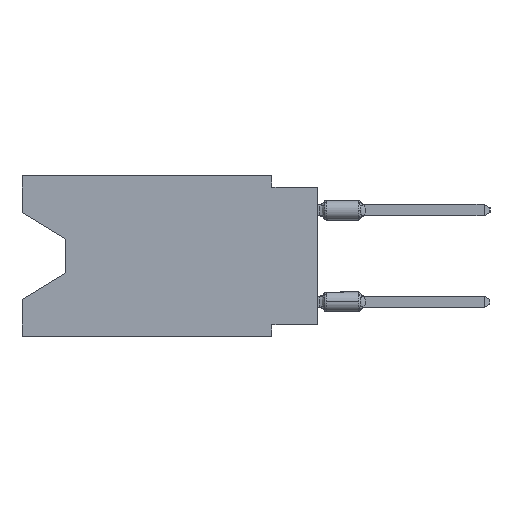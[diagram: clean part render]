
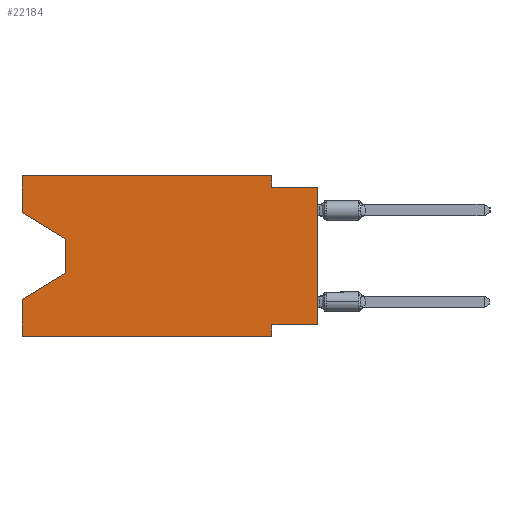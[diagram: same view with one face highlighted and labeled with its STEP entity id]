
A CAD part, left-side view. The second image highlights one B-rep face of the part: STEP entity #22184.
In plain terms, the highlighted planar face has unit normal (-1, 0, 0).
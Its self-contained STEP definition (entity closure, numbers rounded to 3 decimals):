
#291 = VECTOR ( 'NONE', #18357, 1000. ) ;
#392 = VERTEX_POINT ( 'NONE', #48890 ) ;
#420 = CARTESIAN_POINT ( 'NONE',  ( 0., 16.383, -2.038 ) ) ;
#516 = CARTESIAN_POINT ( 'NONE',  ( 0., 2.54, -8.255 ) ) ;
#1358 = EDGE_CURVE ( 'NONE', #392, #31829, #39594, .T. ) ;
#1499 = CARTESIAN_POINT ( 'NONE',  ( 0., 16.383, 0. ) ) ;
#1852 = VECTOR ( 'NONE', #46630, 1000. ) ;
#2166 = CARTESIAN_POINT ( 'NONE',  ( 0., 2.54, -8.89 ) ) ;
#2721 = CARTESIAN_POINT ( 'NONE',  ( 0., 2.54, -8.89 ) ) ;
#3894 = ORIENTED_EDGE ( 'NONE', *, *, #35941, .T. ) ;
#3950 = VECTOR ( 'NONE', #14837, 1000. ) ;
#4140 = CARTESIAN_POINT ( 'NONE',  ( 0., 16.383, 0. ) ) ;
#4143 = CARTESIAN_POINT ( 'NONE',  ( 0., 2.54, 0. ) ) ;
#4407 = CARTESIAN_POINT ( 'NONE',  ( 0., 13.97, -3.505 ) ) ;
#5212 = VECTOR ( 'NONE', #20302, 1000. ) ;
#6039 = DIRECTION ( 'NONE',  ( 0., -1., 0. ) ) ;
#6327 = VERTEX_POINT ( 'NONE', #11023 ) ;
#6406 = CARTESIAN_POINT ( 'NONE',  ( 0., 16.383, -2.038 ) ) ;
#7091 = VECTOR ( 'NONE', #18451, 1000. ) ;
#7501 = EDGE_CURVE ( 'NONE', #31712, #48774, #38444, .T. ) ;
#8876 = VECTOR ( 'NONE', #15474, 1000. ) ;
#8938 = VECTOR ( 'NONE', #41176, 1000. ) ;
#9116 = ORIENTED_EDGE ( 'NONE', *, *, #29129, .T. ) ;
#11023 = CARTESIAN_POINT ( 'NONE',  ( 0., 0., -0.635 ) ) ;
#11464 = FACE_OUTER_BOUND ( 'NONE', #32385, .T. ) ;
#12868 = ORIENTED_EDGE ( 'NONE', *, *, #27389, .T. ) ;
#14200 = CARTESIAN_POINT ( 'NONE',  ( 0., 16.383, 0. ) ) ;
#14381 = LINE ( 'NONE', #41994, #31483 ) ;
#14837 = DIRECTION ( 'NONE',  ( 0., 0., 1. ) ) ;
#15474 = DIRECTION ( 'NONE',  ( 0., 0., -1. ) ) ;
#15889 = DIRECTION ( 'NONE',  ( 1., 0., 0. ) ) ;
#16525 = LINE ( 'NONE', #43897, #22149 ) ;
#16985 = EDGE_CURVE ( 'NONE', #49438, #6327, #14381, .T. ) ;
#17812 = ORIENTED_EDGE ( 'NONE', *, *, #1358, .T. ) ;
#18153 = AXIS2_PLACEMENT_3D ( 'NONE', #4140, #15889, #27371 ) ;
#18357 = DIRECTION ( 'NONE',  ( 0., 0., 1. ) ) ;
#18451 = DIRECTION ( 'NONE',  ( 0., 0., 1. ) ) ;
#18875 = VECTOR ( 'NONE', #50354, 1000. ) ;
#19041 = CARTESIAN_POINT ( 'NONE',  ( 0., 16.383, 0. ) ) ;
#19910 = VERTEX_POINT ( 'NONE', #6406 ) ;
#20302 = DIRECTION ( 'NONE',  ( 0., 0., -1. ) ) ;
#20479 = DIRECTION ( 'NONE',  ( 0., -0.855, -0.519 ) ) ;
#21604 = LINE ( 'NONE', #29696, #8938 ) ;
#22149 = VECTOR ( 'NONE', #40761, 1000. ) ;
#22184 = ADVANCED_FACE ( 'NONE', ( #11464 ), #31798, .F. ) ;
#22480 = ORIENTED_EDGE ( 'NONE', *, *, #46277, .F. ) ;
#22631 = ORIENTED_EDGE ( 'NONE', *, *, #28700, .F. ) ;
#22652 = ORIENTED_EDGE ( 'NONE', *, *, #16985, .F. ) ;
#24172 = CARTESIAN_POINT ( 'NONE',  ( 0., 16.383, -8.89 ) ) ;
#25809 = LINE ( 'NONE', #46136, #3950 ) ;
#26575 = EDGE_CURVE ( 'NONE', #19910, #32272, #49244, .T. ) ;
#26935 = EDGE_CURVE ( 'NONE', #19910, #392, #40306, .T. ) ;
#27371 = DIRECTION ( 'NONE',  ( 0., 0., -1. ) ) ;
#27389 = EDGE_CURVE ( 'NONE', #51131, #48774, #16525, .T. ) ;
#28419 = CARTESIAN_POINT ( 'NONE',  ( 0., 2.54, -0.635 ) ) ;
#28565 = CARTESIAN_POINT ( 'NONE',  ( 0., 16.383, -6.852 ) ) ;
#28700 = EDGE_CURVE ( 'NONE', #32272, #48251, #42776, .T. ) ;
#29129 = EDGE_CURVE ( 'NONE', #31460, #6327, #25809, .T. ) ;
#29696 = CARTESIAN_POINT ( 'NONE',  ( 0., 0., -8.255 ) ) ;
#31098 = EDGE_CURVE ( 'NONE', #51131, #45236, #49905, .T. ) ;
#31460 = VERTEX_POINT ( 'NONE', #42013 ) ;
#31483 = VECTOR ( 'NONE', #6039, 1000. ) ;
#31712 = VERTEX_POINT ( 'NONE', #516 ) ;
#31798 = PLANE ( 'NONE',  #18153 ) ;
#31829 = VERTEX_POINT ( 'NONE', #37796 ) ;
#32272 = VERTEX_POINT ( 'NONE', #1499 ) ;
#32385 = EDGE_LOOP ( 'NONE', ( #50120, #17812, #3894, #47559, #12868, #49596, #43887, #9116, #22652, #22480, #22631, #51454 ) ) ;
#33851 = CARTESIAN_POINT ( 'NONE',  ( 0., 13.97, -5.385 ) ) ;
#35402 = LINE ( 'NONE', #46895, #1852 ) ;
#35836 = EDGE_CURVE ( 'NONE', #31460, #31712, #21604, .T. ) ;
#35941 = EDGE_CURVE ( 'NONE', #31829, #45236, #37003, .T. ) ;
#37003 = LINE ( 'NONE', #33851, #38066 ) ;
#37796 = CARTESIAN_POINT ( 'NONE',  ( 0., 13.97, -5.385 ) ) ;
#38066 = VECTOR ( 'NONE', #49766, 1000. ) ;
#38444 = LINE ( 'NONE', #2721, #8876 ) ;
#38753 = VECTOR ( 'NONE', #20479, 1000. ) ;
#39594 = LINE ( 'NONE', #4407, #5212 ) ;
#40306 = LINE ( 'NONE', #420, #38753 ) ;
#40761 = DIRECTION ( 'NONE',  ( 0., -1., 0. ) ) ;
#41176 = DIRECTION ( 'NONE',  ( 0., 1., 0. ) ) ;
#41994 = CARTESIAN_POINT ( 'NONE',  ( 0., 0., -0.635 ) ) ;
#42013 = CARTESIAN_POINT ( 'NONE',  ( 0., 0., -8.255 ) ) ;
#42776 = LINE ( 'NONE', #19041, #18875 ) ;
#43887 = ORIENTED_EDGE ( 'NONE', *, *, #35836, .F. ) ;
#43897 = CARTESIAN_POINT ( 'NONE',  ( 0., 16.383, -8.89 ) ) ;
#45236 = VERTEX_POINT ( 'NONE', #28565 ) ;
#45833 = CARTESIAN_POINT ( 'NONE',  ( 0., 16.383, 0. ) ) ;
#46136 = CARTESIAN_POINT ( 'NONE',  ( 0., 0., 0. ) ) ;
#46277 = EDGE_CURVE ( 'NONE', #48251, #49438, #35402, .T. ) ;
#46630 = DIRECTION ( 'NONE',  ( 0., 0., -1. ) ) ;
#46895 = CARTESIAN_POINT ( 'NONE',  ( 0., 2.54, 0. ) ) ;
#47559 = ORIENTED_EDGE ( 'NONE', *, *, #31098, .F. ) ;
#48251 = VERTEX_POINT ( 'NONE', #4143 ) ;
#48774 = VERTEX_POINT ( 'NONE', #2166 ) ;
#48890 = CARTESIAN_POINT ( 'NONE',  ( 0., 13.97, -3.505 ) ) ;
#49244 = LINE ( 'NONE', #45833, #7091 ) ;
#49438 = VERTEX_POINT ( 'NONE', #28419 ) ;
#49596 = ORIENTED_EDGE ( 'NONE', *, *, #7501, .F. ) ;
#49766 = DIRECTION ( 'NONE',  ( 0., 0.855, -0.519 ) ) ;
#49905 = LINE ( 'NONE', #14200, #291 ) ;
#50120 = ORIENTED_EDGE ( 'NONE', *, *, #26935, .T. ) ;
#50354 = DIRECTION ( 'NONE',  ( 0., -1., 0. ) ) ;
#51131 = VERTEX_POINT ( 'NONE', #24172 ) ;
#51454 = ORIENTED_EDGE ( 'NONE', *, *, #26575, .F. ) ;
